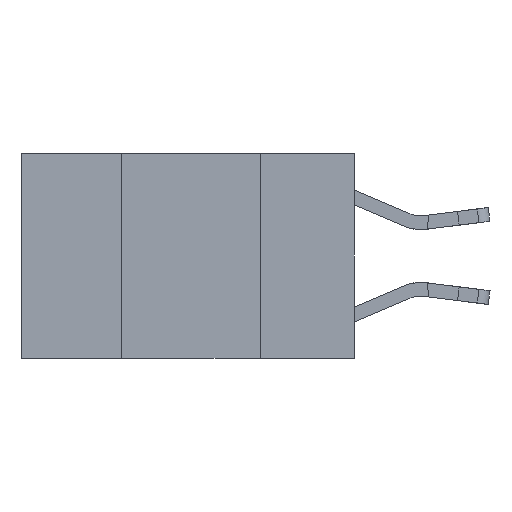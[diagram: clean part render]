
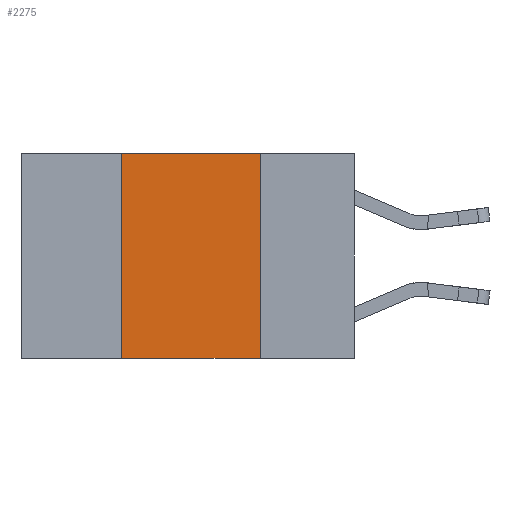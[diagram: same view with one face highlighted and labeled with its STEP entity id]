
A CAD part, left-side view. The second image highlights one B-rep face of the part: STEP entity #2275.
In plain terms, the highlighted planar face has unit normal (-1, 0, 0).
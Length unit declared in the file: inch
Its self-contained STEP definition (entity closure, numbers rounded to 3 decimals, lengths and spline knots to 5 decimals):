
#681 = DIRECTION ( 'NONE',  ( 0., -1., 0. ) ) ;
#1095 = DIRECTION ( 'NONE',  ( 0., 0., -1. ) ) ;
#1201 = ORIENTED_EDGE ( 'NONE', *, *, #9934, .F. ) ;
#1433 = CARTESIAN_POINT ( 'NONE',  ( 0., 0.6, 0. ) ) ;
#1697 = ORIENTED_EDGE ( 'NONE', *, *, #17921, .F. ) ;
#1708 = VECTOR ( 'NONE', #18213, 39.37008 ) ;
#1898 = VECTOR ( 'NONE', #681, 39.37008 ) ;
#2275 = ADVANCED_FACE ( 'NONE', ( #17730 ), #14474, .F. ) ;
#2896 = DIRECTION ( 'NONE',  ( 1., 0., 0. ) ) ;
#3110 = LINE ( 'NONE', #7175, #17635 ) ;
#3266 = LINE ( 'NONE', #18469, #17766 ) ;
#3446 = CARTESIAN_POINT ( 'NONE',  ( 0., 0.17, -0.37 ) ) ;
#3457 = AXIS2_PLACEMENT_3D ( 'NONE', #1433, #2896, #1095 ) ;
#3853 = EDGE_LOOP ( 'NONE', ( #15132, #1201, #1697, #9516 ) ) ;
#4786 = CARTESIAN_POINT ( 'NONE',  ( 0., 0.17, 0. ) ) ;
#5355 = LINE ( 'NONE', #16816, #1708 ) ;
#6024 = EDGE_CURVE ( 'NONE', #13114, #7095, #3110, .T. ) ;
#6703 = CARTESIAN_POINT ( 'NONE',  ( 0., 0.6, 0. ) ) ;
#7095 = VERTEX_POINT ( 'NONE', #3446 ) ;
#7175 = CARTESIAN_POINT ( 'NONE',  ( 0., 0.6, -0.37 ) ) ;
#7305 = VERTEX_POINT ( 'NONE', #17735 ) ;
#9516 = ORIENTED_EDGE ( 'NONE', *, *, #6024, .T. ) ;
#9575 = VERTEX_POINT ( 'NONE', #4786 ) ;
#9704 = LINE ( 'NONE', #6703, #1898 ) ;
#9934 = EDGE_CURVE ( 'NONE', #7305, #9575, #9704, .T. ) ;
#13114 = VERTEX_POINT ( 'NONE', #14590 ) ;
#14117 = DIRECTION ( 'NONE',  ( 0., -1., 0. ) ) ;
#14474 = PLANE ( 'NONE',  #3457 ) ;
#14590 = CARTESIAN_POINT ( 'NONE',  ( 0., 0.42, -0.37 ) ) ;
#15132 = ORIENTED_EDGE ( 'NONE', *, *, #16094, .F. ) ;
#15797 = DIRECTION ( 'NONE',  ( 0., 0., 1. ) ) ;
#16094 = EDGE_CURVE ( 'NONE', #9575, #7095, #5355, .T. ) ;
#16816 = CARTESIAN_POINT ( 'NONE',  ( 0., 0.17, 0. ) ) ;
#17635 = VECTOR ( 'NONE', #14117, 39.37008 ) ;
#17730 = FACE_OUTER_BOUND ( 'NONE', #3853, .T. ) ;
#17735 = CARTESIAN_POINT ( 'NONE',  ( 0., 0.42, 0. ) ) ;
#17766 = VECTOR ( 'NONE', #15797, 39.37008 ) ;
#17921 = EDGE_CURVE ( 'NONE', #13114, #7305, #3266, .T. ) ;
#18213 = DIRECTION ( 'NONE',  ( 0., 0., -1. ) ) ;
#18469 = CARTESIAN_POINT ( 'NONE',  ( 0., 0.42, 0. ) ) ;
